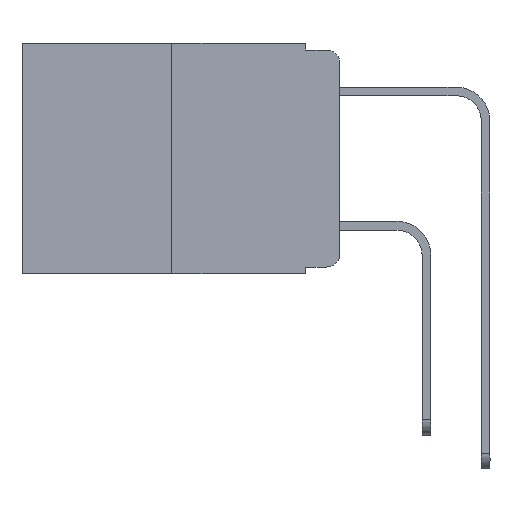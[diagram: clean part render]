
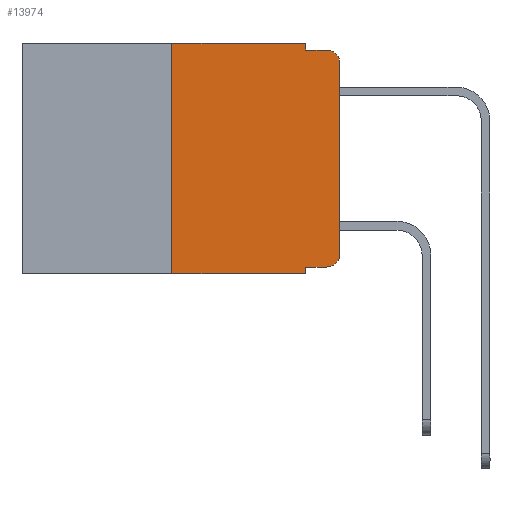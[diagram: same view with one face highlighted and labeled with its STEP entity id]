
A CAD part, left-side view. The second image highlights one B-rep face of the part: STEP entity #13974.
In plain terms, the highlighted planar face has unit normal (-1, 0, 0).
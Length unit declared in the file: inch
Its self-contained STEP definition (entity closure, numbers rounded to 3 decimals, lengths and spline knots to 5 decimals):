
#173 = VECTOR ( 'NONE', #3686, 39.37008 ) ;
#174 = EDGE_CURVE ( 'NONE', #2616, #6240, #10248, .T. ) ;
#590 = ORIENTED_EDGE ( 'NONE', *, *, #6448, .T. ) ;
#950 = LINE ( 'NONE', #11809, #14975 ) ;
#1038 = DIRECTION ( 'NONE',  ( 0., -1., 0. ) ) ;
#1234 = CARTESIAN_POINT ( 'NONE',  ( 0., 0.051, -0.01 ) ) ;
#1311 = EDGE_CURVE ( 'NONE', #2616, #12132, #7704, .T. ) ;
#1350 = FACE_OUTER_BOUND ( 'NONE', #13228, .T. ) ;
#1811 = DIRECTION ( 'NONE',  ( 0., 0., 1. ) ) ;
#2588 = DIRECTION ( 'NONE',  ( 0., 0., -1. ) ) ;
#2616 = VERTEX_POINT ( 'NONE', #6802 ) ;
#3097 = CARTESIAN_POINT ( 'NONE',  ( 0., 0.473, -0.343 ) ) ;
#3112 = CARTESIAN_POINT ( 'NONE',  ( 0., 0.25, 0. ) ) ;
#3613 = DIRECTION ( 'NONE',  ( 0., 0., 1. ) ) ;
#3686 = DIRECTION ( 'NONE',  ( 0., -1., 0. ) ) ;
#3792 = DIRECTION ( 'NONE',  ( 0., -1., 0. ) ) ;
#3837 = LINE ( 'NONE', #4140, #8192 ) ;
#3918 = VECTOR ( 'NONE', #3792, 39.37008 ) ;
#3990 = VECTOR ( 'NONE', #5630, 39.37008 ) ;
#4064 = ORIENTED_EDGE ( 'NONE', *, *, #15245, .F. ) ;
#4140 = CARTESIAN_POINT ( 'NONE',  ( 0., 0.051, -0.333 ) ) ;
#4291 = ORIENTED_EDGE ( 'NONE', *, *, #1311, .F. ) ;
#4981 = DIRECTION ( 'NONE',  ( 0., 0., -1. ) ) ;
#5386 = CARTESIAN_POINT ( 'NONE',  ( 0., 0.02, -0.313 ) ) ;
#5630 = DIRECTION ( 'NONE',  ( 0., 0., -1. ) ) ;
#5906 = CARTESIAN_POINT ( 'NONE',  ( 0., 0., 0. ) ) ;
#6021 = CARTESIAN_POINT ( 'NONE',  ( 0., 0.473, 0. ) ) ;
#6066 = EDGE_CURVE ( 'NONE', #8761, #11148, #12668, .T. ) ;
#6068 = DIRECTION ( 'NONE',  ( -1., 0., 0. ) ) ;
#6240 = VERTEX_POINT ( 'NONE', #9678 ) ;
#6338 = ORIENTED_EDGE ( 'NONE', *, *, #7191, .T. ) ;
#6448 = EDGE_CURVE ( 'NONE', #11148, #11711, #11865, .T. ) ;
#6618 = CIRCLE ( 'NONE', #14123, 0.02 ) ;
#6802 = CARTESIAN_POINT ( 'NONE',  ( 0., 0.25, -0.343 ) ) ;
#6955 = AXIS2_PLACEMENT_3D ( 'NONE', #6021, #13210, #4981 ) ;
#7008 = VERTEX_POINT ( 'NONE', #14405 ) ;
#7191 = EDGE_CURVE ( 'NONE', #7008, #8761, #3837, .T. ) ;
#7704 = LINE ( 'NONE', #8956, #8753 ) ;
#8078 = CARTESIAN_POINT ( 'NONE',  ( 0., 0.051, 0. ) ) ;
#8116 = CARTESIAN_POINT ( 'NONE',  ( 0., 0.02, -0.333 ) ) ;
#8192 = VECTOR ( 'NONE', #12537, 39.37008 ) ;
#8320 = VERTEX_POINT ( 'NONE', #11294 ) ;
#8753 = VECTOR ( 'NONE', #1811, 39.37008 ) ;
#8761 = VERTEX_POINT ( 'NONE', #8116 ) ;
#8810 = ORIENTED_EDGE ( 'NONE', *, *, #6066, .T. ) ;
#8956 = CARTESIAN_POINT ( 'NONE',  ( 0., 0.25, 0. ) ) ;
#9117 = DIRECTION ( 'NONE',  ( 0., 0., -1. ) ) ;
#9565 = EDGE_CURVE ( 'NONE', #11711, #8320, #6618, .T. ) ;
#9678 = CARTESIAN_POINT ( 'NONE',  ( 0., 0.051, -0.343 ) ) ;
#9714 = VERTEX_POINT ( 'NONE', #14085 ) ;
#9943 = ORIENTED_EDGE ( 'NONE', *, *, #11503, .F. ) ;
#10189 = DIRECTION ( 'NONE',  ( 0., 0., -1. ) ) ;
#10248 = LINE ( 'NONE', #3097, #14994 ) ;
#10393 = CARTESIAN_POINT ( 'NONE',  ( 0., 0., -0.313 ) ) ;
#10787 = PLANE ( 'NONE',  #6955 ) ;
#10872 = ORIENTED_EDGE ( 'NONE', *, *, #13517, .F. ) ;
#11148 = VERTEX_POINT ( 'NONE', #10393 ) ;
#11294 = CARTESIAN_POINT ( 'NONE',  ( 0., 0.02, -0.01 ) ) ;
#11319 = LINE ( 'NONE', #14552, #3918 ) ;
#11429 = DIRECTION ( 'NONE',  ( -1., 0., 0. ) ) ;
#11503 = EDGE_CURVE ( 'NONE', #12132, #11825, #11319, .T. ) ;
#11697 = VECTOR ( 'NONE', #3613, 39.37008 ) ;
#11711 = VERTEX_POINT ( 'NONE', #13389 ) ;
#11809 = CARTESIAN_POINT ( 'NONE',  ( 0., 0.051, 0. ) ) ;
#11825 = VERTEX_POINT ( 'NONE', #12378 ) ;
#11854 = LINE ( 'NONE', #1234, #173 ) ;
#11865 = LINE ( 'NONE', #5906, #11697 ) ;
#12132 = VERTEX_POINT ( 'NONE', #3112 ) ;
#12378 = CARTESIAN_POINT ( 'NONE',  ( 0., 0.051, 0. ) ) ;
#12537 = DIRECTION ( 'NONE',  ( 0., -1., 0. ) ) ;
#12668 = CIRCLE ( 'NONE', #14433, 0.02 ) ;
#12726 = ORIENTED_EDGE ( 'NONE', *, *, #14449, .F. ) ;
#13210 = DIRECTION ( 'NONE',  ( 1., 0., 0. ) ) ;
#13228 = EDGE_LOOP ( 'NONE', ( #590, #13341, #10872, #4064, #9943, #4291, #14109, #12726, #6338, #8810 ) ) ;
#13263 = CARTESIAN_POINT ( 'NONE',  ( 0., 0.02, -0.03 ) ) ;
#13341 = ORIENTED_EDGE ( 'NONE', *, *, #9565, .T. ) ;
#13389 = CARTESIAN_POINT ( 'NONE',  ( 0., 0., -0.03 ) ) ;
#13517 = EDGE_CURVE ( 'NONE', #9714, #8320, #11854, .T. ) ;
#13775 = LINE ( 'NONE', #8078, #3990 ) ;
#13974 = ADVANCED_FACE ( 'NONE', ( #1350 ), #10787, .F. ) ;
#14085 = CARTESIAN_POINT ( 'NONE',  ( 0., 0.051, -0.01 ) ) ;
#14109 = ORIENTED_EDGE ( 'NONE', *, *, #174, .T. ) ;
#14123 = AXIS2_PLACEMENT_3D ( 'NONE', #13263, #6068, #2588 ) ;
#14405 = CARTESIAN_POINT ( 'NONE',  ( 0., 0.051, -0.333 ) ) ;
#14433 = AXIS2_PLACEMENT_3D ( 'NONE', #5386, #11429, #10189 ) ;
#14449 = EDGE_CURVE ( 'NONE', #7008, #6240, #950, .T. ) ;
#14552 = CARTESIAN_POINT ( 'NONE',  ( 0., 0.473, 0. ) ) ;
#14975 = VECTOR ( 'NONE', #9117, 39.37008 ) ;
#14994 = VECTOR ( 'NONE', #1038, 39.37008 ) ;
#15245 = EDGE_CURVE ( 'NONE', #11825, #9714, #13775, .T. ) ;
